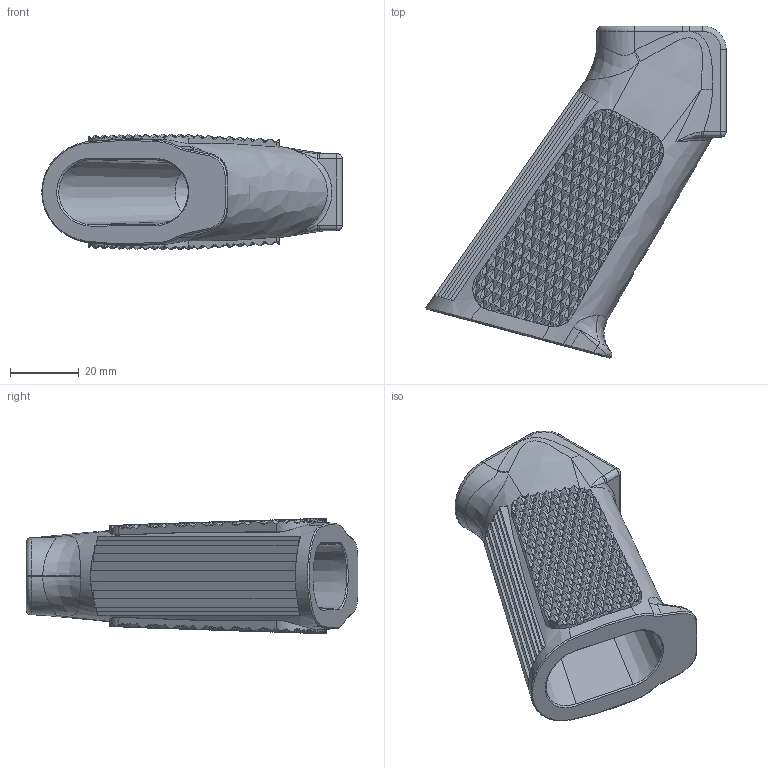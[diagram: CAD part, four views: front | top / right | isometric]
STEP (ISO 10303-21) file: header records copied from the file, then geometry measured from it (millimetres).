
FILE_DESCRIPTION(/* description */ (''),/* implementation_level */ '2;1');
FILE_NAME(/* name */ 'AR GRIP.stp',/* time_stamp */ '2020-08-19T16:02:11+03:00',/* author */ (''),/* organization */ (''),/* preprocessor_version */ 'ST-DEVELOPER v15.2',/* originating_system */ 'Autodesk Translator Framework v2.0.0.5431',/* authorisation */ '');
FILE_SCHEMA (('AUTOMOTIVE_DESIGN { 1 0 10303 214 3 1 1 }'));
Products named in the file (1): MOD9 RETRACT FINAL ASSEMBLY MAGWELL FIXED 2 (production version)
Bounding box: 87.49 x 96.72 x 33.66 mm (x, y, z)
Volume: 67557 mm3; surface area: 23849.7 mm2
Topology: 1 solids, 1 shells, 2430 faces, 5136 edges, 2707 vertices
Faces by surface type: plane 2307, bspline 77, cylinder 35, cone 5, torus 4, sphere 2
Full cylindrical faces by diameter (mm): 3.8 x1, 6.8 x1
Entity records: 66223 total; most frequent: CARTESIAN_POINT 16097, ORIENTED_EDGE 10256, DIRECTION 9868, EDGE_CURVE 5128, LINE 4750, VECTOR 4750, VERTEX_POINT 2705, AXIS2_PLACEMENT_3D 2559
